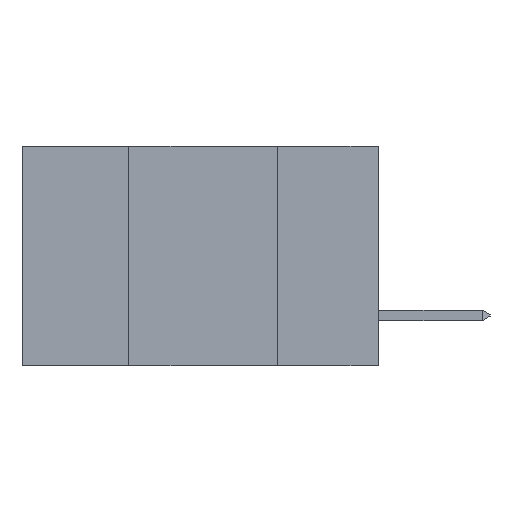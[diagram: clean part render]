
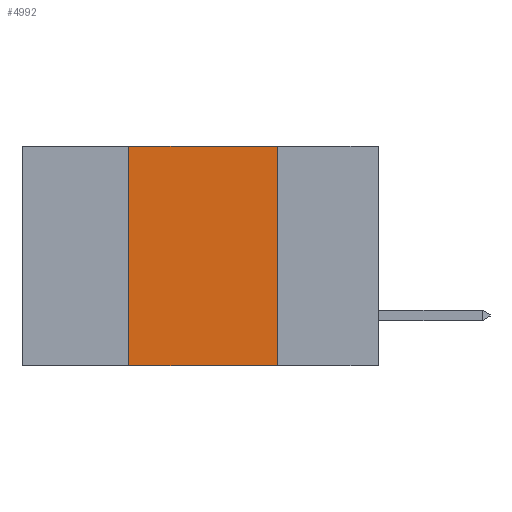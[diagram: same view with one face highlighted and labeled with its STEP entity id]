
A CAD part, left-side view. The second image highlights one B-rep face of the part: STEP entity #4992.
In plain terms, the highlighted planar face has unit normal (-1, 0, 0).
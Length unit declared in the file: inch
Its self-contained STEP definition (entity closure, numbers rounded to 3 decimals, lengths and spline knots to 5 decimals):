
#185 = AXIS2_PLACEMENT_3D ( 'NONE', #15566, #15641, #23673 ) ;
#287 = EDGE_CURVE ( 'NONE', #2367, #23431, #21711, .T. ) ;
#337 = DIRECTION ( 'NONE',  ( 0., 0., -1. ) ) ;
#2367 = VERTEX_POINT ( 'NONE', #12486 ) ;
#2456 = VECTOR ( 'NONE', #15677, 39.37008 ) ;
#2751 = DIRECTION ( 'NONE',  ( 0., 0., 1. ) ) ;
#4365 = VERTEX_POINT ( 'NONE', #18054 ) ;
#4992 = ADVANCED_FACE ( 'NONE', ( #19609 ), #14960, .F. ) ;
#7122 = VECTOR ( 'NONE', #2751, 39.37008 ) ;
#7123 = CARTESIAN_POINT ( 'NONE',  ( 0., 0.17, -0.37 ) ) ;
#8287 = LINE ( 'NONE', #14763, #12670 ) ;
#9876 = VERTEX_POINT ( 'NONE', #7123 ) ;
#10101 = CARTESIAN_POINT ( 'NONE',  ( 0., 0.42, 0. ) ) ;
#12486 = CARTESIAN_POINT ( 'NONE',  ( 0., 0.42, 0. ) ) ;
#12670 = VECTOR ( 'NONE', #24084, 39.37008 ) ;
#12809 = EDGE_CURVE ( 'NONE', #4365, #9876, #8287, .T. ) ;
#13135 = LINE ( 'NONE', #20783, #22546 ) ;
#13320 = ORIENTED_EDGE ( 'NONE', *, *, #12809, .T. ) ;
#14339 = EDGE_CURVE ( 'NONE', #4365, #2367, #22036, .T. ) ;
#14567 = ORIENTED_EDGE ( 'NONE', *, *, #15573, .F. ) ;
#14763 = CARTESIAN_POINT ( 'NONE',  ( 0., 0.6, -0.37 ) ) ;
#14876 = EDGE_LOOP ( 'NONE', ( #14567, #15843, #17162, #13320 ) ) ;
#14960 = PLANE ( 'NONE',  #185 ) ;
#15566 = CARTESIAN_POINT ( 'NONE',  ( 0., 0.6, 0. ) ) ;
#15573 = EDGE_CURVE ( 'NONE', #23431, #9876, #13135, .T. ) ;
#15641 = DIRECTION ( 'NONE',  ( 1., 0., 0. ) ) ;
#15677 = DIRECTION ( 'NONE',  ( 0., -1., 0. ) ) ;
#15843 = ORIENTED_EDGE ( 'NONE', *, *, #287, .F. ) ;
#17162 = ORIENTED_EDGE ( 'NONE', *, *, #14339, .F. ) ;
#18054 = CARTESIAN_POINT ( 'NONE',  ( 0., 0.42, -0.37 ) ) ;
#18975 = CARTESIAN_POINT ( 'NONE',  ( 0., 0.6, 0. ) ) ;
#19609 = FACE_OUTER_BOUND ( 'NONE', #14876, .T. ) ;
#20783 = CARTESIAN_POINT ( 'NONE',  ( 0., 0.17, 0. ) ) ;
#21711 = LINE ( 'NONE', #18975, #2456 ) ;
#21794 = CARTESIAN_POINT ( 'NONE',  ( 0., 0.17, 0. ) ) ;
#22036 = LINE ( 'NONE', #10101, #7122 ) ;
#22546 = VECTOR ( 'NONE', #337, 39.37008 ) ;
#23431 = VERTEX_POINT ( 'NONE', #21794 ) ;
#23673 = DIRECTION ( 'NONE',  ( 0., 0., -1. ) ) ;
#24084 = DIRECTION ( 'NONE',  ( 0., -1., 0. ) ) ;
